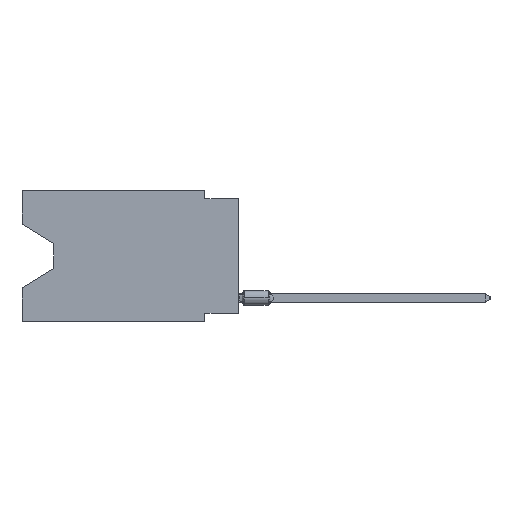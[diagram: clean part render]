
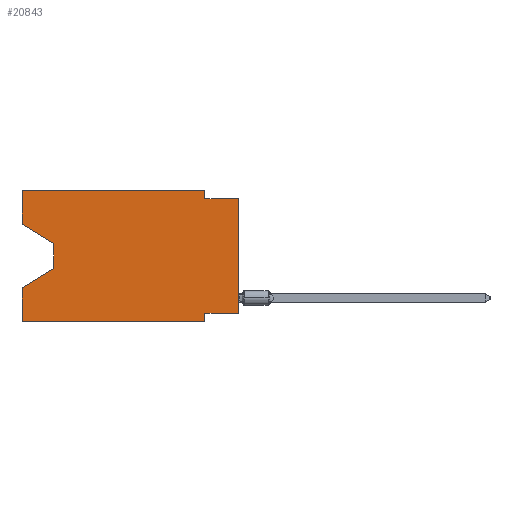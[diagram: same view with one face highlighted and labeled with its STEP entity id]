
A CAD part, left-side view. The second image highlights one B-rep face of the part: STEP entity #20843.
In plain terms, the highlighted planar face has unit normal (-1, 0, 0).
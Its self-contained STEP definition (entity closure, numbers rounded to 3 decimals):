
#87 = VECTOR ( 'NONE', #40380, 1000. ) ;
#487 = VECTOR ( 'NONE', #19720, 1000. ) ;
#1516 = AXIS2_PLACEMENT_3D ( 'NONE', #5605, #23884, #47891 ) ;
#1627 = CARTESIAN_POINT ( 'NONE',  ( 0., 16.383, 0. ) ) ;
#2641 = VERTEX_POINT ( 'NONE', #46279 ) ;
#2994 = DIRECTION ( 'NONE',  ( 0., 0., -1. ) ) ;
#3923 = DIRECTION ( 'NONE',  ( 0., -1., 0. ) ) ;
#5605 = CARTESIAN_POINT ( 'NONE',  ( 0., 16.383, 0. ) ) ;
#5682 = LINE ( 'NONE', #45611, #40338 ) ;
#6239 = EDGE_CURVE ( 'NONE', #46184, #50082, #29900, .T. ) ;
#6402 = CARTESIAN_POINT ( 'NONE',  ( 0., 0., 0. ) ) ;
#6426 = LINE ( 'NONE', #38528, #38864 ) ;
#7587 = CARTESIAN_POINT ( 'NONE',  ( 0., 2.54, -0.635 ) ) ;
#9126 = EDGE_CURVE ( 'NONE', #46184, #55112, #57676, .T. ) ;
#10391 = FACE_OUTER_BOUND ( 'NONE', #41579, .T. ) ;
#10530 = ORIENTED_EDGE ( 'NONE', *, *, #33713, .F. ) ;
#10641 = VERTEX_POINT ( 'NONE', #40310 ) ;
#11517 = CARTESIAN_POINT ( 'NONE',  ( 0., 13.97, -4.013 ) ) ;
#12136 = ORIENTED_EDGE ( 'NONE', *, *, #31445, .T. ) ;
#12420 = VERTEX_POINT ( 'NONE', #34529 ) ;
#12754 = LINE ( 'NONE', #30754, #27103 ) ;
#13063 = DIRECTION ( 'NONE',  ( 0., -1., 0. ) ) ;
#13293 = ORIENTED_EDGE ( 'NONE', *, *, #6239, .T. ) ;
#13592 = ORIENTED_EDGE ( 'NONE', *, *, #48954, .T. ) ;
#13897 = CARTESIAN_POINT ( 'NONE',  ( 0., 2.54, -9.906 ) ) ;
#17133 = LINE ( 'NONE', #31829, #50081 ) ;
#18391 = VECTOR ( 'NONE', #23692, 1000. ) ;
#18584 = DIRECTION ( 'NONE',  ( 0., 0., -1. ) ) ;
#18729 = EDGE_CURVE ( 'NONE', #2641, #55112, #6426, .T. ) ;
#19720 = DIRECTION ( 'NONE',  ( 0., -1., 0. ) ) ;
#20740 = CARTESIAN_POINT ( 'NONE',  ( 0., 2.54, 0. ) ) ;
#20843 = ADVANCED_FACE ( 'NONE', ( #10391 ), #38600, .F. ) ;
#21161 = EDGE_CURVE ( 'NONE', #39428, #48428, #28557, .T. ) ;
#22420 = VERTEX_POINT ( 'NONE', #56333 ) ;
#23692 = DIRECTION ( 'NONE',  ( 0., -0.855, -0.519 ) ) ;
#23884 = DIRECTION ( 'NONE',  ( 1., 0., 0. ) ) ;
#27103 = VECTOR ( 'NONE', #13063, 1000. ) ;
#27478 = VECTOR ( 'NONE', #39971, 1000. ) ;
#28557 = LINE ( 'NONE', #42366, #32337 ) ;
#29375 = ORIENTED_EDGE ( 'NONE', *, *, #46955, .F. ) ;
#29735 = ORIENTED_EDGE ( 'NONE', *, *, #54124, .T. ) ;
#29900 = LINE ( 'NONE', #37747, #487 ) ;
#30365 = LINE ( 'NONE', #39675, #27478 ) ;
#30754 = CARTESIAN_POINT ( 'NONE',  ( 0., 16.383, 0. ) ) ;
#30762 = LINE ( 'NONE', #54206, #87 ) ;
#31445 = EDGE_CURVE ( 'NONE', #39428, #47823, #52018, .T. ) ;
#31829 = CARTESIAN_POINT ( 'NONE',  ( 0., 0., -0.635 ) ) ;
#32337 = VECTOR ( 'NONE', #43243, 1000. ) ;
#32526 = DIRECTION ( 'NONE',  ( 0., 0.855, -0.519 ) ) ;
#33537 = ORIENTED_EDGE ( 'NONE', *, *, #48144, .F. ) ;
#33713 = EDGE_CURVE ( 'NONE', #48428, #50082, #30365, .T. ) ;
#33995 = DIRECTION ( 'NONE',  ( 0., 0., 1. ) ) ;
#34267 = VECTOR ( 'NONE', #42474, 1000. ) ;
#34529 = CARTESIAN_POINT ( 'NONE',  ( 0., 16.383, -2.546 ) ) ;
#36324 = LINE ( 'NONE', #49831, #18391 ) ;
#37590 = ORIENTED_EDGE ( 'NONE', *, *, #57633, .F. ) ;
#37747 = CARTESIAN_POINT ( 'NONE',  ( 0., 16.383, -9.906 ) ) ;
#37999 = ORIENTED_EDGE ( 'NONE', *, *, #9126, .F. ) ;
#38149 = CARTESIAN_POINT ( 'NONE',  ( 0., 2.54, -9.271 ) ) ;
#38528 = CARTESIAN_POINT ( 'NONE',  ( 0., 13.97, -5.893 ) ) ;
#38600 = PLANE ( 'NONE',  #1516 ) ;
#38864 = VECTOR ( 'NONE', #32526, 1000. ) ;
#39428 = VERTEX_POINT ( 'NONE', #40619 ) ;
#39675 = CARTESIAN_POINT ( 'NONE',  ( 0., 2.54, -9.906 ) ) ;
#39971 = DIRECTION ( 'NONE',  ( 0., 0., -1. ) ) ;
#40310 = CARTESIAN_POINT ( 'NONE',  ( 0., 16.383, 0. ) ) ;
#40338 = VECTOR ( 'NONE', #18584, 1000. ) ;
#40380 = DIRECTION ( 'NONE',  ( 0., 0., 1. ) ) ;
#40619 = CARTESIAN_POINT ( 'NONE',  ( 0., 0., -9.271 ) ) ;
#41322 = VECTOR ( 'NONE', #2994, 1000. ) ;
#41579 = EDGE_LOOP ( 'NONE', ( #13592, #29735, #56354, #37999, #13293, #10530, #55904, #12136, #37590, #51339, #29375, #33537 ) ) ;
#42366 = CARTESIAN_POINT ( 'NONE',  ( 0., 0., -9.271 ) ) ;
#42474 = DIRECTION ( 'NONE',  ( 0., 0., 1. ) ) ;
#43243 = DIRECTION ( 'NONE',  ( 0., 1., 0. ) ) ;
#44131 = LINE ( 'NONE', #20740, #41322 ) ;
#45611 = CARTESIAN_POINT ( 'NONE',  ( 0., 13.97, -4.013 ) ) ;
#46184 = VERTEX_POINT ( 'NONE', #49534 ) ;
#46279 = CARTESIAN_POINT ( 'NONE',  ( 0., 13.97, -5.893 ) ) ;
#46955 = EDGE_CURVE ( 'NONE', #10641, #22420, #12754, .T. ) ;
#47823 = VERTEX_POINT ( 'NONE', #58773 ) ;
#47891 = DIRECTION ( 'NONE',  ( 0., 0., -1. ) ) ;
#48144 = EDGE_CURVE ( 'NONE', #12420, #10641, #30762, .T. ) ;
#48371 = VERTEX_POINT ( 'NONE', #11517 ) ;
#48428 = VERTEX_POINT ( 'NONE', #38149 ) ;
#48954 = EDGE_CURVE ( 'NONE', #12420, #48371, #36324, .T. ) ;
#49384 = VECTOR ( 'NONE', #33995, 1000. ) ;
#49534 = CARTESIAN_POINT ( 'NONE',  ( 0., 16.383, -9.906 ) ) ;
#49831 = CARTESIAN_POINT ( 'NONE',  ( 0., 16.383, -2.546 ) ) ;
#50081 = VECTOR ( 'NONE', #3923, 1000. ) ;
#50082 = VERTEX_POINT ( 'NONE', #13897 ) ;
#51160 = CARTESIAN_POINT ( 'NONE',  ( 0., 16.383, -7.36 ) ) ;
#51339 = ORIENTED_EDGE ( 'NONE', *, *, #55673, .F. ) ;
#52018 = LINE ( 'NONE', #6402, #49384 ) ;
#54124 = EDGE_CURVE ( 'NONE', #48371, #2641, #5682, .T. ) ;
#54206 = CARTESIAN_POINT ( 'NONE',  ( 0., 16.383, 0. ) ) ;
#55112 = VERTEX_POINT ( 'NONE', #51160 ) ;
#55241 = VERTEX_POINT ( 'NONE', #7587 ) ;
#55673 = EDGE_CURVE ( 'NONE', #22420, #55241, #44131, .T. ) ;
#55904 = ORIENTED_EDGE ( 'NONE', *, *, #21161, .F. ) ;
#56333 = CARTESIAN_POINT ( 'NONE',  ( 0., 2.54, 0. ) ) ;
#56354 = ORIENTED_EDGE ( 'NONE', *, *, #18729, .T. ) ;
#57633 = EDGE_CURVE ( 'NONE', #55241, #47823, #17133, .T. ) ;
#57676 = LINE ( 'NONE', #1627, #34267 ) ;
#58773 = CARTESIAN_POINT ( 'NONE',  ( 0., 0., -0.635 ) ) ;
